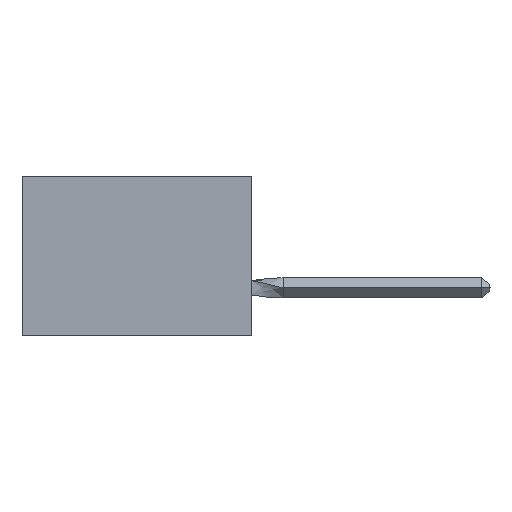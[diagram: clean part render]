
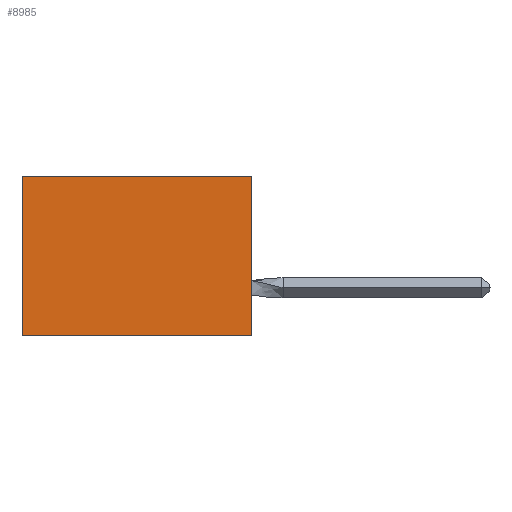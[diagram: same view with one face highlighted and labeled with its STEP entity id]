
A CAD part, left-side view. The second image highlights one B-rep face of the part: STEP entity #8985.
In plain terms, the highlighted planar face has unit normal (-1, 0, 0).
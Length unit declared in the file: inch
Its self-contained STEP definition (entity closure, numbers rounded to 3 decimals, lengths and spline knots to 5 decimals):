
#347 = VERTEX_POINT ( 'NONE', #13997 ) ;
#1477 = DIRECTION ( 'NONE',  ( 1., 0., 0. ) ) ;
#1766 = AXIS2_PLACEMENT_3D ( 'NONE', #21551, #1477, #23298 ) ;
#2402 = ORIENTED_EDGE ( 'NONE', *, *, #13136, .T. ) ;
#2446 = VERTEX_POINT ( 'NONE', #9295 ) ;
#3476 = LINE ( 'NONE', #12907, #17642 ) ;
#4225 = LINE ( 'NONE', #18164, #15551 ) ;
#4234 = DIRECTION ( 'NONE',  ( 0., 1., 0. ) ) ;
#4482 = EDGE_CURVE ( 'NONE', #347, #21464, #10055, .T. ) ;
#5519 = ORIENTED_EDGE ( 'NONE', *, *, #6570, .F. ) ;
#5734 = DIRECTION ( 'NONE',  ( 0., 0., -1. ) ) ;
#6346 = EDGE_CURVE ( 'NONE', #2446, #21464, #9672, .T. ) ;
#6570 = EDGE_CURVE ( 'NONE', #20954, #2446, #3476, .T. ) ;
#6580 = CARTESIAN_POINT ( 'NONE',  ( 0.305, 0., 0. ) ) ;
#6876 = CARTESIAN_POINT ( 'NONE',  ( 0.305, 0.72, -0.5 ) ) ;
#7369 = DIRECTION ( 'NONE',  ( 0., 1., 0. ) ) ;
#8985 = ADVANCED_FACE ( 'NONE', ( #16632 ), #10631, .F. ) ;
#9295 = CARTESIAN_POINT ( 'NONE',  ( 0.305, 0., -0.5 ) ) ;
#9672 = LINE ( 'NONE', #13635, #19675 ) ;
#10055 = LINE ( 'NONE', #6876, #23450 ) ;
#10631 = PLANE ( 'NONE',  #1766 ) ;
#12907 = CARTESIAN_POINT ( 'NONE',  ( 0.305, 0., -0.5 ) ) ;
#13136 = EDGE_CURVE ( 'NONE', #20954, #347, #4225, .T. ) ;
#13635 = CARTESIAN_POINT ( 'NONE',  ( 0.305, 0., -0.5 ) ) ;
#13997 = CARTESIAN_POINT ( 'NONE',  ( 0.305, 0.72, 0. ) ) ;
#15551 = VECTOR ( 'NONE', #7369, 39.37008 ) ;
#15738 = ORIENTED_EDGE ( 'NONE', *, *, #6346, .F. ) ;
#16560 = CARTESIAN_POINT ( 'NONE',  ( 0.305, 0.72, -0.5 ) ) ;
#16632 = FACE_OUTER_BOUND ( 'NONE', #20959, .T. ) ;
#17642 = VECTOR ( 'NONE', #5734, 39.37008 ) ;
#18164 = CARTESIAN_POINT ( 'NONE',  ( 0.305, 0., 0. ) ) ;
#19497 = DIRECTION ( 'NONE',  ( 0., 0., -1. ) ) ;
#19675 = VECTOR ( 'NONE', #4234, 39.37008 ) ;
#20954 = VERTEX_POINT ( 'NONE', #6580 ) ;
#20959 = EDGE_LOOP ( 'NONE', ( #21181, #15738, #5519, #2402 ) ) ;
#21181 = ORIENTED_EDGE ( 'NONE', *, *, #4482, .T. ) ;
#21464 = VERTEX_POINT ( 'NONE', #16560 ) ;
#21551 = CARTESIAN_POINT ( 'NONE',  ( 0.305, 0., -0.5 ) ) ;
#23298 = DIRECTION ( 'NONE',  ( 0., 0., -1. ) ) ;
#23450 = VECTOR ( 'NONE', #19497, 39.37008 ) ;
